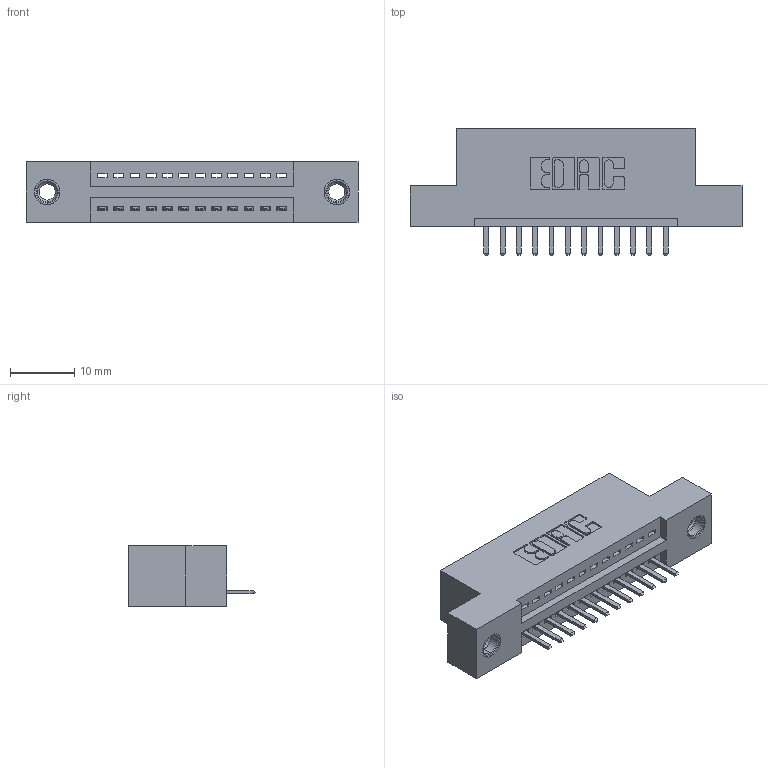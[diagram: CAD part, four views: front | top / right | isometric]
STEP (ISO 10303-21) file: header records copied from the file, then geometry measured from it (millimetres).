
FILE_DESCRIPTION (( 'STEP AP203' ), '1' );
FILE_NAME ('345-012-520-107.STEP', '2019-10-04T00:57:43', ( '' ), ( '' ), 'SwSTEP 2.0', 'SolidWorks 2016', '' );
FILE_SCHEMA (( 'CONFIG_CONTROL_DESIGN' ));
Length unit declared in the file: inch
Products named in the file (4): 345-250-001_345-250-005-103; 345-292-001_345-293-120; 345 Part_Flush Mounting Lugs - 0.156 Dia-TI; 345-012-520-107
Assembly tree (15 placements, depth 2):
  345-012-520-107
    345 Part_Flush Mounting Lugs - 0.156 Dia-TI
    345-292-001_345-293-120  x12
    345-250-001_345-250-005-103  x2
Bounding box: 51.69 x 19.68 x 9.4 mm (x, y, z)
Volume: 4615.7 mm3; surface area: 5645.7 mm2
Topology: 15 solids, 15 shells, 930 faces, 2685 edges, 1750 vertices
Faces by surface type: plane 616, cylinder 298, cone 12, torus 4
Entity records: 14370 total; most frequent: CARTESIAN_POINT 2483, ORIENTED_EDGE 2410, DIRECTION 2227, EDGE_CURVE 1205, VECTOR 1001, LINE 1001, VERTEX_POINT 796, AXIS2_PLACEMENT_3D 613
